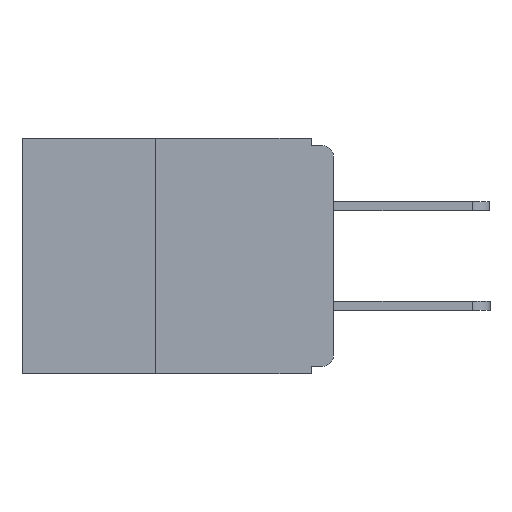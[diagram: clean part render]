
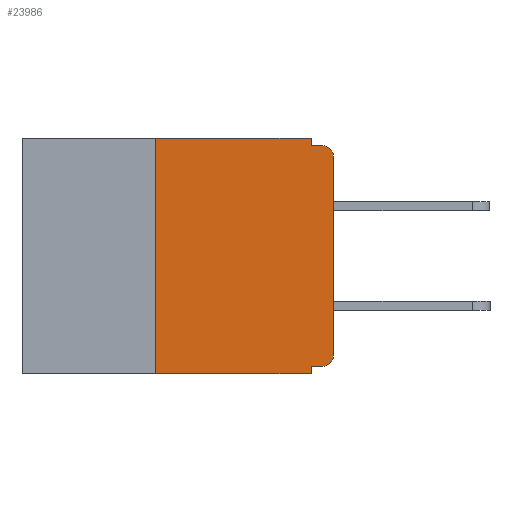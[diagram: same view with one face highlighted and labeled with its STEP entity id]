
A CAD part, left-side view. The second image highlights one B-rep face of the part: STEP entity #23986.
In plain terms, the highlighted planar face has unit normal (-1, 0, 0).
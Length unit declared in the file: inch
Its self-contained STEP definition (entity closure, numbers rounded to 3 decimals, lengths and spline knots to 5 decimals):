
#498 = DIRECTION ( 'NONE',  ( 0., 0., 1. ) ) ;
#575 = VERTEX_POINT ( 'NONE', #26716 ) ;
#1545 = CARTESIAN_POINT ( 'NONE',  ( 0., 0.015, -0.025 ) ) ;
#1564 = LINE ( 'NONE', #13766, #24305 ) ;
#1581 = VERTEX_POINT ( 'NONE', #21301 ) ;
#1860 = DIRECTION ( 'NONE',  ( 0., 0., -1. ) ) ;
#2125 = CARTESIAN_POINT ( 'NONE',  ( 0., 0.015, -0.305 ) ) ;
#2424 = AXIS2_PLACEMENT_3D ( 'NONE', #1545, #17007, #3775 ) ;
#2538 = CARTESIAN_POINT ( 'NONE',  ( 0., 0.437, 0. ) ) ;
#2797 = VECTOR ( 'NONE', #5880, 39.37008 ) ;
#3330 = DIRECTION ( 'NONE',  ( 0., -1., 0. ) ) ;
#3685 = VECTOR ( 'NONE', #25555, 39.37008 ) ;
#3775 = DIRECTION ( 'NONE',  ( 0., 0., -1. ) ) ;
#3876 = VERTEX_POINT ( 'NONE', #13298 ) ;
#4357 = DIRECTION ( 'NONE',  ( 0., 0., -1. ) ) ;
#4882 = DIRECTION ( 'NONE',  ( 0., 0., -1. ) ) ;
#5355 = DIRECTION ( 'NONE',  ( 0., 0., -1. ) ) ;
#5384 = VERTEX_POINT ( 'NONE', #6092 ) ;
#5880 = DIRECTION ( 'NONE',  ( 0., -1., 0. ) ) ;
#6092 = CARTESIAN_POINT ( 'NONE',  ( 0., 0., -0.305 ) ) ;
#6427 = CARTESIAN_POINT ( 'NONE',  ( 0., 0.015, -0.01 ) ) ;
#6560 = EDGE_CURVE ( 'NONE', #14734, #21092, #18209, .T. ) ;
#7020 = DIRECTION ( 'NONE',  ( 0., 1., 0. ) ) ;
#7124 = CARTESIAN_POINT ( 'NONE',  ( 0., 0.25, 0. ) ) ;
#7448 = AXIS2_PLACEMENT_3D ( 'NONE', #2538, #18079, #4882 ) ;
#8170 = VERTEX_POINT ( 'NONE', #19779 ) ;
#8792 = VECTOR ( 'NONE', #3330, 39.37008 ) ;
#8867 = CARTESIAN_POINT ( 'NONE',  ( 0., 0.031, -0.01 ) ) ;
#9776 = EDGE_CURVE ( 'NONE', #5384, #14734, #26300, .T. ) ;
#9954 = EDGE_CURVE ( 'NONE', #1581, #5384, #15772, .T. ) ;
#10822 = VERTEX_POINT ( 'NONE', #24090 ) ;
#11482 = VECTOR ( 'NONE', #7020, 39.37008 ) ;
#11511 = PLANE ( 'NONE',  #7448 ) ;
#12537 = CARTESIAN_POINT ( 'NONE',  ( 0., 0., -0.01 ) ) ;
#12654 = EDGE_LOOP ( 'NONE', ( #21750, #21914, #22338, #23426, #23703, #24511, #24843, #25662, #26333, #27154 ) ) ;
#12876 = CARTESIAN_POINT ( 'NONE',  ( 0., 0.437, 0. ) ) ;
#13298 = CARTESIAN_POINT ( 'NONE',  ( 0., 0.25, -0.33 ) ) ;
#13766 = CARTESIAN_POINT ( 'NONE',  ( 0., 0.25, -0.33 ) ) ;
#14552 = LINE ( 'NONE', #12537, #2797 ) ;
#14613 = LINE ( 'NONE', #18686, #8792 ) ;
#14734 = VERTEX_POINT ( 'NONE', #21247 ) ;
#15079 = DIRECTION ( 'NONE',  ( 0., -1., 0. ) ) ;
#15745 = CARTESIAN_POINT ( 'NONE',  ( 0., 0., -0.32 ) ) ;
#15772 = CIRCLE ( 'NONE', #25842, 0.015 ) ;
#15870 = EDGE_CURVE ( 'NONE', #3876, #575, #14613, .T. ) ;
#16073 = EDGE_CURVE ( 'NONE', #8170, #575, #26504, .T. ) ;
#16181 = VERTEX_POINT ( 'NONE', #8867 ) ;
#16803 = CARTESIAN_POINT ( 'NONE',  ( 0., 0., 0. ) ) ;
#17007 = DIRECTION ( 'NONE',  ( -1., 0., 0. ) ) ;
#17258 = LINE ( 'NONE', #15745, #11482 ) ;
#17327 = EDGE_CURVE ( 'NONE', #28134, #10822, #23432, .T. ) ;
#17546 = EDGE_CURVE ( 'NONE', #1581, #8170, #17258, .T. ) ;
#17565 = DIRECTION ( 'NONE',  ( -1., 0., 0. ) ) ;
#18079 = DIRECTION ( 'NONE',  ( 1., 0., 0. ) ) ;
#18192 = LINE ( 'NONE', #20785, #18873 ) ;
#18209 = CIRCLE ( 'NONE', #2424, 0.015 ) ;
#18682 = FACE_OUTER_BOUND ( 'NONE', #12654, .T. ) ;
#18686 = CARTESIAN_POINT ( 'NONE',  ( 0., 0.437, -0.33 ) ) ;
#18873 = VECTOR ( 'NONE', #5355, 39.37008 ) ;
#19429 = CARTESIAN_POINT ( 'NONE',  ( 0., 0.031, -0.33 ) ) ;
#19478 = EDGE_CURVE ( 'NONE', #10822, #16181, #18192, .T. ) ;
#19779 = CARTESIAN_POINT ( 'NONE',  ( 0., 0.031, -0.32 ) ) ;
#20785 = CARTESIAN_POINT ( 'NONE',  ( 0., 0.031, 0. ) ) ;
#20832 = VECTOR ( 'NONE', #1860, 39.37008 ) ;
#21092 = VERTEX_POINT ( 'NONE', #6427 ) ;
#21191 = EDGE_CURVE ( 'NONE', #3876, #28134, #1564, .T. ) ;
#21247 = CARTESIAN_POINT ( 'NONE',  ( 0., 0., -0.025 ) ) ;
#21301 = CARTESIAN_POINT ( 'NONE',  ( 0., 0.015, -0.32 ) ) ;
#21750 = ORIENTED_EDGE ( 'NONE', *, *, #9776, .T. ) ;
#21914 = ORIENTED_EDGE ( 'NONE', *, *, #6560, .T. ) ;
#22338 = ORIENTED_EDGE ( 'NONE', *, *, #23658, .F. ) ;
#22767 = VECTOR ( 'NONE', #15079, 39.37008 ) ;
#23426 = ORIENTED_EDGE ( 'NONE', *, *, #19478, .F. ) ;
#23432 = LINE ( 'NONE', #12876, #22767 ) ;
#23658 = EDGE_CURVE ( 'NONE', #16181, #21092, #14552, .T. ) ;
#23703 = ORIENTED_EDGE ( 'NONE', *, *, #17327, .F. ) ;
#23986 = ADVANCED_FACE ( 'NONE', ( #18682 ), #11511, .F. ) ;
#24090 = CARTESIAN_POINT ( 'NONE',  ( 0., 0.031, 0. ) ) ;
#24305 = VECTOR ( 'NONE', #498, 39.37008 ) ;
#24511 = ORIENTED_EDGE ( 'NONE', *, *, #21191, .F. ) ;
#24843 = ORIENTED_EDGE ( 'NONE', *, *, #15870, .T. ) ;
#25555 = DIRECTION ( 'NONE',  ( 0., 0., 1. ) ) ;
#25662 = ORIENTED_EDGE ( 'NONE', *, *, #16073, .F. ) ;
#25842 = AXIS2_PLACEMENT_3D ( 'NONE', #2125, #17565, #4357 ) ;
#26300 = LINE ( 'NONE', #16803, #3685 ) ;
#26333 = ORIENTED_EDGE ( 'NONE', *, *, #17546, .F. ) ;
#26504 = LINE ( 'NONE', #19429, #20832 ) ;
#26716 = CARTESIAN_POINT ( 'NONE',  ( 0., 0.031, -0.33 ) ) ;
#27154 = ORIENTED_EDGE ( 'NONE', *, *, #9954, .T. ) ;
#28134 = VERTEX_POINT ( 'NONE', #7124 ) ;
